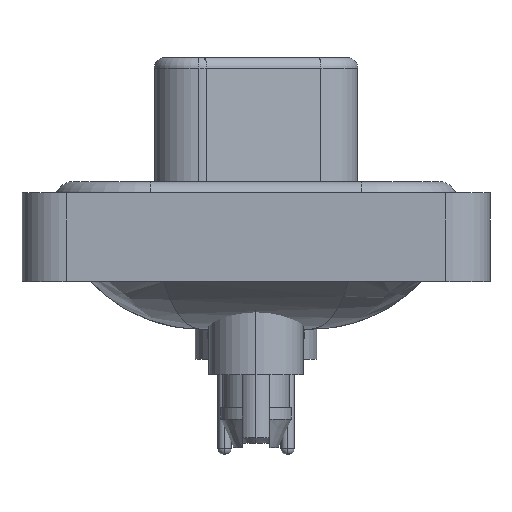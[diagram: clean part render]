
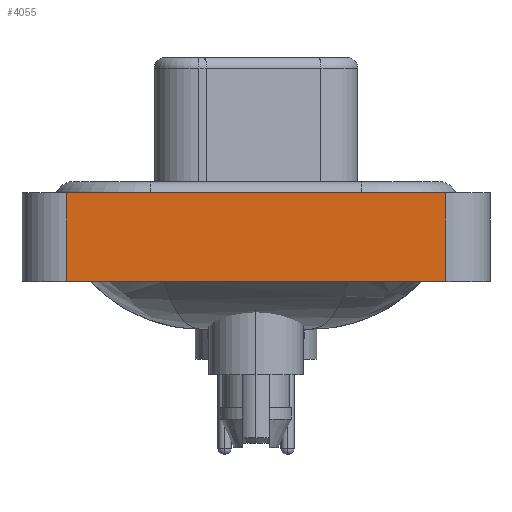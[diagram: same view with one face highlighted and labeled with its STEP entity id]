
A CAD part, left-side view. The second image highlights one B-rep face of the part: STEP entity #4055.
In plain terms, the highlighted planar face has unit normal (-1, 0, 0).
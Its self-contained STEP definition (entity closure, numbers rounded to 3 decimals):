
#837 = CARTESIAN_POINT ( 'NONE',  ( -7.35, 8.55, -3.6 ) ) ;
#1093 = ORIENTED_EDGE ( 'NONE', *, *, #28212, .T. ) ;
#1771 = VECTOR ( 'NONE', #9260, 1000. ) ;
#2137 = VERTEX_POINT ( 'NONE', #4947 ) ;
#2838 = EDGE_CURVE ( 'NONE', #20301, #17853, #10663, .T. ) ;
#3576 = ORIENTED_EDGE ( 'NONE', *, *, #10979, .F. ) ;
#4055 = ADVANCED_FACE ( 'NONE', ( #19800 ), #17166, .T. ) ;
#4123 = DIRECTION ( 'NONE',  ( -1., 0., 0. ) ) ;
#4384 = VECTOR ( 'NONE', #24035, 1000. ) ;
#4947 = CARTESIAN_POINT ( 'NONE',  ( -7.35, 8.55, -3.6 ) ) ;
#5371 = EDGE_CURVE ( 'NONE', #2137, #17032, #17254, .T. ) ;
#5706 = AXIS2_PLACEMENT_3D ( 'NONE', #26168, #4123, #19662 ) ;
#6324 = CARTESIAN_POINT ( 'NONE',  ( -7.35, -8.55, -3.6 ) ) ;
#7622 = ORIENTED_EDGE ( 'NONE', *, *, #5371, .T. ) ;
#9260 = DIRECTION ( 'NONE',  ( 0., 0., 1. ) ) ;
#9407 = CARTESIAN_POINT ( 'NONE',  ( -7.35, -8.55, 0.4 ) ) ;
#9441 = CARTESIAN_POINT ( 'NONE',  ( -7.35, -8.55, -3.6 ) ) ;
#9590 = DIRECTION ( 'NONE',  ( 0., 0., 1. ) ) ;
#9971 = CARTESIAN_POINT ( 'NONE',  ( -7.35, 8.55, 0.4 ) ) ;
#10663 = LINE ( 'NONE', #28678, #15096 ) ;
#10979 = EDGE_CURVE ( 'NONE', #2137, #20301, #20634, .T. ) ;
#14608 = LINE ( 'NONE', #9441, #22767 ) ;
#15017 = CARTESIAN_POINT ( 'NONE',  ( -7.35, -8.55, -3.6 ) ) ;
#15096 = VECTOR ( 'NONE', #19833, 1000. ) ;
#17032 = VERTEX_POINT ( 'NONE', #6324 ) ;
#17166 = PLANE ( 'NONE',  #5706 ) ;
#17254 = LINE ( 'NONE', #15017, #4384 ) ;
#17853 = VERTEX_POINT ( 'NONE', #9407 ) ;
#18890 = EDGE_LOOP ( 'NONE', ( #1093, #23926, #3576, #7622 ) ) ;
#19662 = DIRECTION ( 'NONE',  ( 0., 0., 1. ) ) ;
#19800 = FACE_OUTER_BOUND ( 'NONE', #18890, .T. ) ;
#19833 = DIRECTION ( 'NONE',  ( 0., -1., 0. ) ) ;
#20301 = VERTEX_POINT ( 'NONE', #9971 ) ;
#20634 = LINE ( 'NONE', #837, #1771 ) ;
#22767 = VECTOR ( 'NONE', #9590, 1000. ) ;
#23926 = ORIENTED_EDGE ( 'NONE', *, *, #2838, .F. ) ;
#24035 = DIRECTION ( 'NONE',  ( 0., -1., 0. ) ) ;
#26168 = CARTESIAN_POINT ( 'NONE',  ( -7.35, -8.55, -3.6 ) ) ;
#28212 = EDGE_CURVE ( 'NONE', #17032, #17853, #14608, .T. ) ;
#28678 = CARTESIAN_POINT ( 'NONE',  ( -7.35, -8.55, 0.4 ) ) ;
